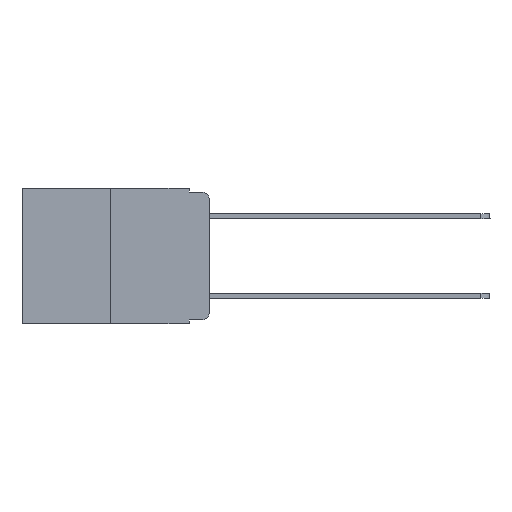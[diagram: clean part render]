
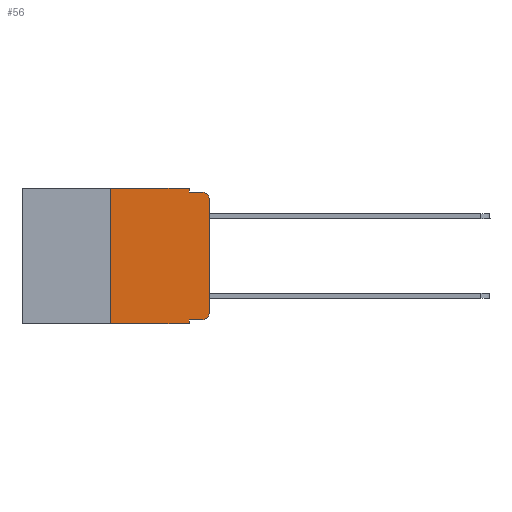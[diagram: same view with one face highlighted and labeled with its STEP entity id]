
A CAD part, left-side view. The second image highlights one B-rep face of the part: STEP entity #56.
In plain terms, the highlighted planar face has unit normal (-1, 0, 0).
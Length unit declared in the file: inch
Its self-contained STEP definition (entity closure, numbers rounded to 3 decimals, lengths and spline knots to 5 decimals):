
#56 = ADVANCED_FACE ( 'NONE', ( #15951 ), #3390, .F. ) ;
#106 = LINE ( 'NONE', #11789, #7462 ) ;
#143 = EDGE_CURVE ( 'NONE', #6726, #6393, #2136, .T. ) ;
#535 = CARTESIAN_POINT ( 'NONE',  ( 0., 0.051, -0.333 ) ) ;
#854 = CIRCLE ( 'NONE', #17566, 0.02 ) ;
#940 = LINE ( 'NONE', #17921, #18840 ) ;
#1003 = LINE ( 'NONE', #15626, #12653 ) ;
#1417 = CARTESIAN_POINT ( 'NONE',  ( 0., 0.02, -0.333 ) ) ;
#1766 = DIRECTION ( 'NONE',  ( 0., 0., 1. ) ) ;
#2136 = LINE ( 'NONE', #8896, #21085 ) ;
#2190 = EDGE_CURVE ( 'NONE', #19773, #9212, #106, .T. ) ;
#2430 = EDGE_CURVE ( 'NONE', #17690, #17502, #11493, .T. ) ;
#2673 = LINE ( 'NONE', #5873, #11348 ) ;
#2958 = AXIS2_PLACEMENT_3D ( 'NONE', #6288, #4681, #16975 ) ;
#3347 = VECTOR ( 'NONE', #13744, 39.37008 ) ;
#3390 = PLANE ( 'NONE',  #4795 ) ;
#3910 = VERTEX_POINT ( 'NONE', #18541 ) ;
#4106 = ORIENTED_EDGE ( 'NONE', *, *, #143, .T. ) ;
#4171 = DIRECTION ( 'NONE',  ( 0., -1., 0. ) ) ;
#4204 = VERTEX_POINT ( 'NONE', #19588 ) ;
#4375 = EDGE_CURVE ( 'NONE', #4204, #18980, #2673, .T. ) ;
#4681 = DIRECTION ( 'NONE',  ( -1., 0., 0. ) ) ;
#4795 = AXIS2_PLACEMENT_3D ( 'NONE', #20976, #10591, #6913 ) ;
#4896 = ORIENTED_EDGE ( 'NONE', *, *, #11904, .T. ) ;
#5115 = DIRECTION ( 'NONE',  ( 0., 0., 1. ) ) ;
#5162 = VERTEX_POINT ( 'NONE', #12052 ) ;
#5199 = EDGE_CURVE ( 'NONE', #4204, #3910, #1003, .T. ) ;
#5741 = CARTESIAN_POINT ( 'NONE',  ( 0., 0., -0.03 ) ) ;
#5873 = CARTESIAN_POINT ( 'NONE',  ( 0., 0.473, -0.343 ) ) ;
#6288 = CARTESIAN_POINT ( 'NONE',  ( 0., 0.02, -0.313 ) ) ;
#6393 = VERTEX_POINT ( 'NONE', #1417 ) ;
#6726 = VERTEX_POINT ( 'NONE', #535 ) ;
#6913 = DIRECTION ( 'NONE',  ( 0., 0., -1. ) ) ;
#7403 = EDGE_CURVE ( 'NONE', #3910, #17690, #940, .T. ) ;
#7462 = VECTOR ( 'NONE', #5115, 39.37008 ) ;
#7592 = ORIENTED_EDGE ( 'NONE', *, *, #16459, .T. ) ;
#7627 = CARTESIAN_POINT ( 'NONE',  ( 0., 0.051, -0.01 ) ) ;
#7719 = DIRECTION ( 'NONE',  ( 0., -1., 0. ) ) ;
#7762 = ORIENTED_EDGE ( 'NONE', *, *, #2190, .T. ) ;
#8221 = CARTESIAN_POINT ( 'NONE',  ( 0., 0.02, -0.03 ) ) ;
#8565 = ORIENTED_EDGE ( 'NONE', *, *, #2430, .F. ) ;
#8760 = DIRECTION ( 'NONE',  ( 0., -1., 0. ) ) ;
#8896 = CARTESIAN_POINT ( 'NONE',  ( 0., 0.051, -0.333 ) ) ;
#9050 = CARTESIAN_POINT ( 'NONE',  ( 0., 0.051, 0. ) ) ;
#9212 = VERTEX_POINT ( 'NONE', #5741 ) ;
#9770 = VECTOR ( 'NONE', #18275, 39.37008 ) ;
#9911 = EDGE_CURVE ( 'NONE', #17502, #5162, #21663, .T. ) ;
#10591 = DIRECTION ( 'NONE',  ( 1., 0., 0. ) ) ;
#11348 = VECTOR ( 'NONE', #4171, 39.37008 ) ;
#11493 = LINE ( 'NONE', #9050, #17721 ) ;
#11695 = DIRECTION ( 'NONE',  ( -1., 0., 0. ) ) ;
#11789 = CARTESIAN_POINT ( 'NONE',  ( 0., 0., 0. ) ) ;
#11904 = EDGE_CURVE ( 'NONE', #9212, #5162, #854, .T. ) ;
#12052 = CARTESIAN_POINT ( 'NONE',  ( 0., 0.02, -0.01 ) ) ;
#12231 = ORIENTED_EDGE ( 'NONE', *, *, #5199, .F. ) ;
#12250 = EDGE_LOOP ( 'NONE', ( #7762, #4896, #13192, #8565, #16067, #12231, #18545, #21991, #4106, #7592 ) ) ;
#12653 = VECTOR ( 'NONE', #1766, 39.37008 ) ;
#12916 = CARTESIAN_POINT ( 'NONE',  ( 0., 0.051, -0.01 ) ) ;
#13192 = ORIENTED_EDGE ( 'NONE', *, *, #9911, .F. ) ;
#13368 = CARTESIAN_POINT ( 'NONE',  ( 0., 0.051, 0. ) ) ;
#13451 = DIRECTION ( 'NONE',  ( 0., 0., -1. ) ) ;
#13673 = LINE ( 'NONE', #18809, #3347 ) ;
#13744 = DIRECTION ( 'NONE',  ( 0., 0., -1. ) ) ;
#14447 = CARTESIAN_POINT ( 'NONE',  ( 0., 0., -0.313 ) ) ;
#15626 = CARTESIAN_POINT ( 'NONE',  ( 0., 0.25, 0. ) ) ;
#15951 = FACE_OUTER_BOUND ( 'NONE', #12250, .T. ) ;
#16067 = ORIENTED_EDGE ( 'NONE', *, *, #7403, .F. ) ;
#16459 = EDGE_CURVE ( 'NONE', #6393, #19773, #21545, .T. ) ;
#16939 = CARTESIAN_POINT ( 'NONE',  ( 0., 0.051, -0.343 ) ) ;
#16975 = DIRECTION ( 'NONE',  ( 0., 0., -1. ) ) ;
#17502 = VERTEX_POINT ( 'NONE', #7627 ) ;
#17566 = AXIS2_PLACEMENT_3D ( 'NONE', #8221, #11695, #13451 ) ;
#17690 = VERTEX_POINT ( 'NONE', #13368 ) ;
#17721 = VECTOR ( 'NONE', #21084, 39.37008 ) ;
#17807 = EDGE_CURVE ( 'NONE', #6726, #18980, #13673, .T. ) ;
#17921 = CARTESIAN_POINT ( 'NONE',  ( 0., 0.473, 0. ) ) ;
#18275 = DIRECTION ( 'NONE',  ( 0., -1., 0. ) ) ;
#18541 = CARTESIAN_POINT ( 'NONE',  ( 0., 0.25, 0. ) ) ;
#18545 = ORIENTED_EDGE ( 'NONE', *, *, #4375, .T. ) ;
#18809 = CARTESIAN_POINT ( 'NONE',  ( 0., 0.051, 0. ) ) ;
#18840 = VECTOR ( 'NONE', #7719, 39.37008 ) ;
#18980 = VERTEX_POINT ( 'NONE', #16939 ) ;
#19588 = CARTESIAN_POINT ( 'NONE',  ( 0., 0.25, -0.343 ) ) ;
#19773 = VERTEX_POINT ( 'NONE', #14447 ) ;
#20976 = CARTESIAN_POINT ( 'NONE',  ( 0., 0.473, 0. ) ) ;
#21084 = DIRECTION ( 'NONE',  ( 0., 0., -1. ) ) ;
#21085 = VECTOR ( 'NONE', #8760, 39.37008 ) ;
#21545 = CIRCLE ( 'NONE', #2958, 0.02 ) ;
#21663 = LINE ( 'NONE', #12916, #9770 ) ;
#21991 = ORIENTED_EDGE ( 'NONE', *, *, #17807, .F. ) ;
